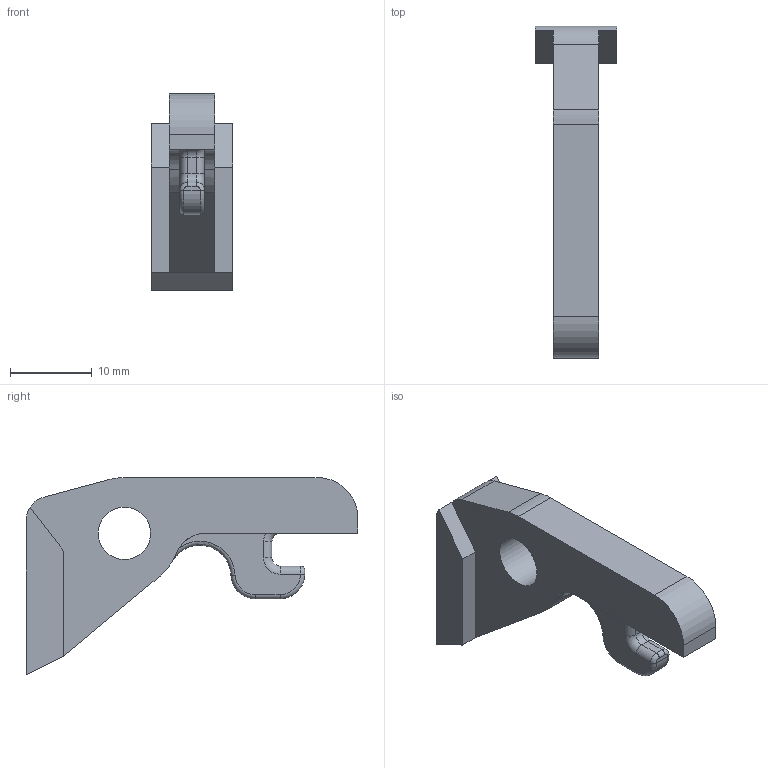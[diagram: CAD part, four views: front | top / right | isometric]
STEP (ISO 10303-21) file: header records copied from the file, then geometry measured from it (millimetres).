
FILE_DESCRIPTION((''),'2;1');
FILE_NAME('PM522Sear2.stp','2015-10-01T18:17:27',('JamesRPatrick'),(''),'Autodesk Inventor 2012','Autodesk Inventor 2012','');
FILE_SCHEMA(('AUTOMOTIVE_DESIGN { 1 0 10303 214 1 1 1 1 }'));
Length unit declared in the file: millimetre
Products named in the file (1): PM522Sear2
Bounding box: 10 x 40.5 x 24.03 mm (x, y, z)
Volume: 2900.9 mm3; surface area: 1953.3 mm2
Topology: 1 solids, 1 shells, 52 faces, 130 edges, 80 vertices
Faces by surface type: plane 21, cylinder 19, torus 10, bspline 2
Full cylindrical faces by diameter (mm): 6.4 x1
Entity records: 1745 total; most frequent: CARTESIAN_POINT 452, DIRECTION 281, ORIENTED_EDGE 258, EDGE_CURVE 129, AXIS2_PLACEMENT_3D 107, VERTEX_POINT 80, VECTOR 67, LINE 67
